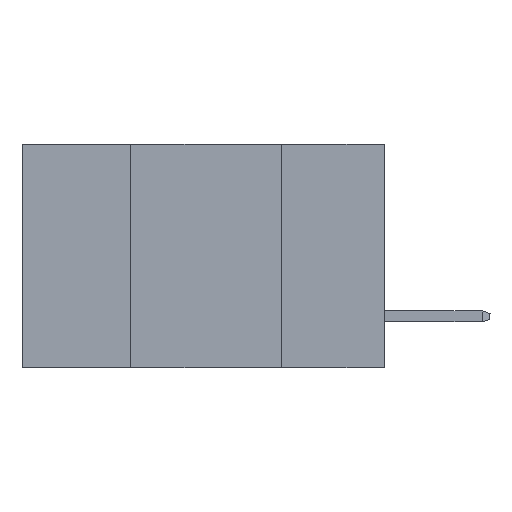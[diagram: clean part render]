
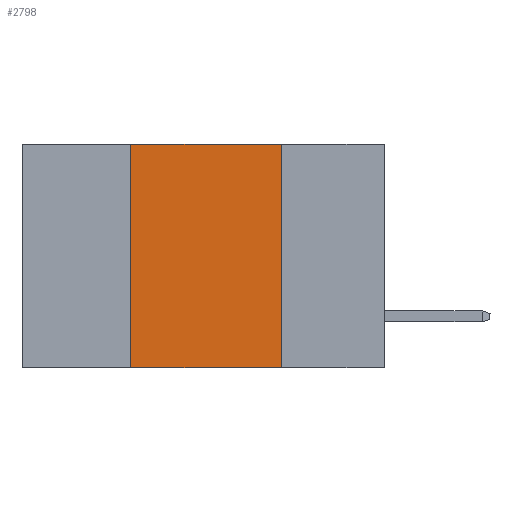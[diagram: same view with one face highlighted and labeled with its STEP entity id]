
A CAD part, left-side view. The second image highlights one B-rep face of the part: STEP entity #2798.
In plain terms, the highlighted planar face has unit normal (-1, 0, 0).
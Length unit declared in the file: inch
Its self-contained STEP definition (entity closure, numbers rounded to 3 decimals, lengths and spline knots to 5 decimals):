
#122 = EDGE_CURVE ( 'NONE', #9245, #4513, #4537, .T. ) ;
#472 = DIRECTION ( 'NONE',  ( 0., -1., 0. ) ) ;
#892 = EDGE_CURVE ( 'NONE', #12392, #4542, #9759, .T. ) ;
#1022 = CARTESIAN_POINT ( 'NONE',  ( 0., 0.17, -0.37 ) ) ;
#1049 = CARTESIAN_POINT ( 'NONE',  ( 0., 0.6, -0.37 ) ) ;
#2798 = ADVANCED_FACE ( 'NONE', ( #3497 ), #5493, .F. ) ;
#2811 = ORIENTED_EDGE ( 'NONE', *, *, #892, .F. ) ;
#3489 = CARTESIAN_POINT ( 'NONE',  ( 0., 0.42, -0.37 ) ) ;
#3497 = FACE_OUTER_BOUND ( 'NONE', #9649, .T. ) ;
#4107 = VECTOR ( 'NONE', #472, 39.37008 ) ;
#4513 = VERTEX_POINT ( 'NONE', #5358 ) ;
#4537 = LINE ( 'NONE', #3489, #10497 ) ;
#4542 = VERTEX_POINT ( 'NONE', #7529 ) ;
#4553 = CARTESIAN_POINT ( 'NONE',  ( 0., 0.42, -0.37 ) ) ;
#5358 = CARTESIAN_POINT ( 'NONE',  ( 0., 0.42, 0. ) ) ;
#5370 = DIRECTION ( 'NONE',  ( 0., 0., -1. ) ) ;
#5456 = EDGE_CURVE ( 'NONE', #4513, #12392, #11041, .T. ) ;
#5493 = PLANE ( 'NONE',  #10833 ) ;
#5637 = VECTOR ( 'NONE', #10610, 39.37008 ) ;
#5970 = LINE ( 'NONE', #1049, #11924 ) ;
#6452 = CARTESIAN_POINT ( 'NONE',  ( 0., 0.6, 0. ) ) ;
#6836 = EDGE_CURVE ( 'NONE', #9245, #4542, #5970, .T. ) ;
#7529 = CARTESIAN_POINT ( 'NONE',  ( 0., 0.17, -0.37 ) ) ;
#8053 = ORIENTED_EDGE ( 'NONE', *, *, #5456, .F. ) ;
#8307 = DIRECTION ( 'NONE',  ( 0., 0., 1. ) ) ;
#8912 = DIRECTION ( 'NONE',  ( 0., -1., 0. ) ) ;
#9236 = ORIENTED_EDGE ( 'NONE', *, *, #6836, .T. ) ;
#9245 = VERTEX_POINT ( 'NONE', #4553 ) ;
#9649 = EDGE_LOOP ( 'NONE', ( #2811, #8053, #11215, #9236 ) ) ;
#9759 = LINE ( 'NONE', #1022, #5637 ) ;
#10337 = CARTESIAN_POINT ( 'NONE',  ( 0., 0.6, 0. ) ) ;
#10497 = VECTOR ( 'NONE', #8307, 39.37008 ) ;
#10610 = DIRECTION ( 'NONE',  ( 0., 0., -1. ) ) ;
#10833 = AXIS2_PLACEMENT_3D ( 'NONE', #6452, #12381, #5370 ) ;
#11041 = LINE ( 'NONE', #10337, #4107 ) ;
#11215 = ORIENTED_EDGE ( 'NONE', *, *, #122, .F. ) ;
#11924 = VECTOR ( 'NONE', #8912, 39.37008 ) ;
#12060 = CARTESIAN_POINT ( 'NONE',  ( 0., 0.17, 0. ) ) ;
#12381 = DIRECTION ( 'NONE',  ( 1., 0., 0. ) ) ;
#12392 = VERTEX_POINT ( 'NONE', #12060 ) ;
